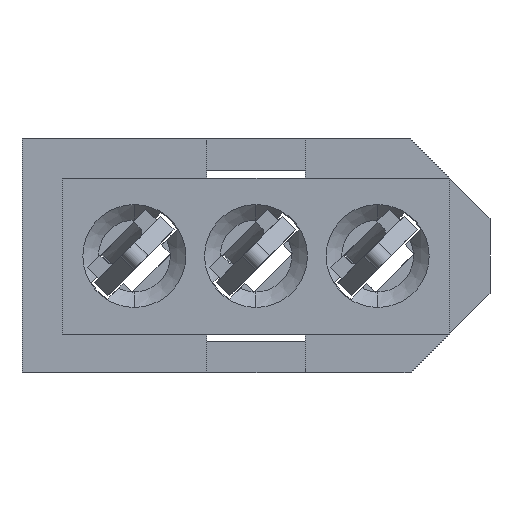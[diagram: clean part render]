
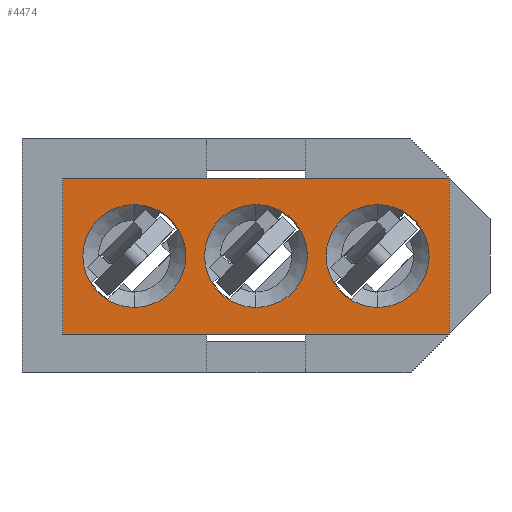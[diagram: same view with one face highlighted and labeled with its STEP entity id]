
A CAD part, front view. The second image highlights one B-rep face of the part: STEP entity #4474.
In plain terms, the highlighted planar face has unit normal (0, -1, 0).
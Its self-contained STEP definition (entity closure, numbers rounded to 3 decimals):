
#9 = EDGE_LOOP ( 'NONE', ( #2040, #771, #2001, #3821 ) ) ;
#65 = CARTESIAN_POINT ( 'NONE',  ( 0., -12.7, 0. ) ) ;
#254 = CARTESIAN_POINT ( 'NONE',  ( 3.962, -12.7, 1.676 ) ) ;
#388 = LINE ( 'NONE', #1455, #5583 ) ;
#542 = LINE ( 'NONE', #3797, #3066 ) ;
#565 = DIRECTION ( 'NONE',  ( 0., 0., 1. ) ) ;
#586 = AXIS2_PLACEMENT_3D ( 'NONE', #2626, #593, #5675 ) ;
#593 = DIRECTION ( 'NONE',  ( 0., 1., 0. ) ) ;
#771 = ORIENTED_EDGE ( 'NONE', *, *, #4602, .F. ) ;
#879 = DIRECTION ( 'NONE',  ( 1., 0., 0. ) ) ;
#964 = CARTESIAN_POINT ( 'NONE',  ( -2.324, -12.7, -2.54 ) ) ;
#1041 = FACE_BOUND ( 'NONE', #6220, .T. ) ;
#1257 = LINE ( 'NONE', #3853, #3906 ) ;
#1378 = AXIS2_PLACEMENT_3D ( 'NONE', #65, #4117, #565 ) ;
#1455 = CARTESIAN_POINT ( 'NONE',  ( -2.324, -12.7, -2.54 ) ) ;
#1521 = VERTEX_POINT ( 'NONE', #4332 ) ;
#1573 = EDGE_LOOP ( 'NONE', ( #3069, #2738 ) ) ;
#1607 = LINE ( 'NONE', #964, #5761 ) ;
#1710 = AXIS2_PLACEMENT_3D ( 'NONE', #2483, #3422, #2882 ) ;
#1718 = DIRECTION ( 'NONE',  ( 0., 0., 1. ) ) ;
#1769 = CIRCLE ( 'NONE', #2635, 1.676 ) ;
#1939 = PLANE ( 'NONE',  #6029 ) ;
#1948 = DIRECTION ( 'NONE',  ( -1., 0., 0. ) ) ;
#2001 = ORIENTED_EDGE ( 'NONE', *, *, #5042, .F. ) ;
#2040 = ORIENTED_EDGE ( 'NONE', *, *, #6297, .F. ) ;
#2057 = EDGE_LOOP ( 'NONE', ( #5653, #4884 ) ) ;
#2153 = FACE_BOUND ( 'NONE', #2057, .T. ) ;
#2242 = CIRCLE ( 'NONE', #2863, 1.676 ) ;
#2424 = DIRECTION ( 'NONE',  ( 0., 0., 1. ) ) ;
#2483 = CARTESIAN_POINT ( 'NONE',  ( 7.925, -12.7, 0. ) ) ;
#2559 = CARTESIAN_POINT ( 'NONE',  ( -2.324, -12.7, -2.54 ) ) ;
#2589 = EDGE_CURVE ( 'NONE', #5866, #1521, #1769, .T. ) ;
#2626 = CARTESIAN_POINT ( 'NONE',  ( 0., -12.7, 0. ) ) ;
#2635 = AXIS2_PLACEMENT_3D ( 'NONE', #3576, #3041, #4999 ) ;
#2738 = ORIENTED_EDGE ( 'NONE', *, *, #6352, .T. ) ;
#2773 = EDGE_CURVE ( 'NONE', #4012, #5973, #2242, .T. ) ;
#2781 = CARTESIAN_POINT ( 'NONE',  ( 0., -12.7, 1.676 ) ) ;
#2792 = CARTESIAN_POINT ( 'NONE',  ( 10.249, -12.7, -2.54 ) ) ;
#2863 = AXIS2_PLACEMENT_3D ( 'NONE', #5123, #5626, #1718 ) ;
#2882 = DIRECTION ( 'NONE',  ( 0., 0., 1. ) ) ;
#2941 = DIRECTION ( 'NONE',  ( 0., 0., 1. ) ) ;
#2960 = CARTESIAN_POINT ( 'NONE',  ( 3.962, -12.7, 0. ) ) ;
#2969 = VERTEX_POINT ( 'NONE', #4285 ) ;
#3041 = DIRECTION ( 'NONE',  ( 0., 1., 0. ) ) ;
#3066 = VECTOR ( 'NONE', #5298, 1000. ) ;
#3069 = ORIENTED_EDGE ( 'NONE', *, *, #5404, .T. ) ;
#3141 = ORIENTED_EDGE ( 'NONE', *, *, #3747, .T. ) ;
#3422 = DIRECTION ( 'NONE',  ( 0., 1., 0. ) ) ;
#3473 = CARTESIAN_POINT ( 'NONE',  ( 0., -12.7, -1.676 ) ) ;
#3576 = CARTESIAN_POINT ( 'NONE',  ( 7.925, -12.7, 0. ) ) ;
#3747 = EDGE_CURVE ( 'NONE', #1521, #5866, #4100, .T. ) ;
#3797 = CARTESIAN_POINT ( 'NONE',  ( 10.249, -12.7, -2.54 ) ) ;
#3821 = ORIENTED_EDGE ( 'NONE', *, *, #5600, .F. ) ;
#3853 = CARTESIAN_POINT ( 'NONE',  ( -2.324, -12.7, 2.54 ) ) ;
#3906 = VECTOR ( 'NONE', #879, 1000. ) ;
#4012 = VERTEX_POINT ( 'NONE', #254 ) ;
#4049 = DIRECTION ( 'NONE',  ( 0., 0., 1. ) ) ;
#4079 = CARTESIAN_POINT ( 'NONE',  ( 7.925, -12.7, 1.676 ) ) ;
#4100 = CIRCLE ( 'NONE', #1710, 1.676 ) ;
#4104 = VERTEX_POINT ( 'NONE', #2792 ) ;
#4117 = DIRECTION ( 'NONE',  ( 0., 1., 0. ) ) ;
#4285 = CARTESIAN_POINT ( 'NONE',  ( -2.324, -12.7, 2.54 ) ) ;
#4332 = CARTESIAN_POINT ( 'NONE',  ( 7.925, -12.7, -1.676 ) ) ;
#4474 = ADVANCED_FACE ( 'NONE', ( #1041, #2153, #5050, #4888 ), #1939, .F. ) ;
#4602 = EDGE_CURVE ( 'NONE', #4104, #6424, #388, .T. ) ;
#4883 = CARTESIAN_POINT ( 'NONE',  ( 0., -12.7, 0. ) ) ;
#4884 = ORIENTED_EDGE ( 'NONE', *, *, #6214, .T. ) ;
#4888 = FACE_OUTER_BOUND ( 'NONE', #9, .T. ) ;
#4999 = DIRECTION ( 'NONE',  ( 0., 0., 1. ) ) ;
#5042 = EDGE_CURVE ( 'NONE', #6289, #4104, #542, .T. ) ;
#5050 = FACE_BOUND ( 'NONE', #1573, .T. ) ;
#5123 = CARTESIAN_POINT ( 'NONE',  ( 3.962, -12.7, 0. ) ) ;
#5183 = VERTEX_POINT ( 'NONE', #2781 ) ;
#5217 = CIRCLE ( 'NONE', #5309, 1.676 ) ;
#5298 = DIRECTION ( 'NONE',  ( 0., 0., -1. ) ) ;
#5309 = AXIS2_PLACEMENT_3D ( 'NONE', #2960, #5506, #2941 ) ;
#5331 = CIRCLE ( 'NONE', #586, 1.676 ) ;
#5382 = DIRECTION ( 'NONE',  ( 0., 1., 0. ) ) ;
#5404 = EDGE_CURVE ( 'NONE', #5183, #6196, #5331, .T. ) ;
#5506 = DIRECTION ( 'NONE',  ( 0., 1., 0. ) ) ;
#5583 = VECTOR ( 'NONE', #1948, 1000. ) ;
#5597 = CARTESIAN_POINT ( 'NONE',  ( 10.249, -12.7, 2.54 ) ) ;
#5600 = EDGE_CURVE ( 'NONE', #2969, #6289, #1257, .T. ) ;
#5626 = DIRECTION ( 'NONE',  ( 0., 1., 0. ) ) ;
#5647 = CARTESIAN_POINT ( 'NONE',  ( 3.962, -12.7, -1.676 ) ) ;
#5653 = ORIENTED_EDGE ( 'NONE', *, *, #2773, .T. ) ;
#5675 = DIRECTION ( 'NONE',  ( 0., 0., 1. ) ) ;
#5761 = VECTOR ( 'NONE', #4049, 1000. ) ;
#5866 = VERTEX_POINT ( 'NONE', #4079 ) ;
#5973 = VERTEX_POINT ( 'NONE', #5647 ) ;
#5979 = ORIENTED_EDGE ( 'NONE', *, *, #2589, .T. ) ;
#6029 = AXIS2_PLACEMENT_3D ( 'NONE', #4883, #5382, #2424 ) ;
#6156 = CIRCLE ( 'NONE', #1378, 1.676 ) ;
#6196 = VERTEX_POINT ( 'NONE', #3473 ) ;
#6214 = EDGE_CURVE ( 'NONE', #5973, #4012, #5217, .T. ) ;
#6220 = EDGE_LOOP ( 'NONE', ( #5979, #3141 ) ) ;
#6289 = VERTEX_POINT ( 'NONE', #5597 ) ;
#6297 = EDGE_CURVE ( 'NONE', #6424, #2969, #1607, .T. ) ;
#6352 = EDGE_CURVE ( 'NONE', #6196, #5183, #6156, .T. ) ;
#6424 = VERTEX_POINT ( 'NONE', #2559 ) ;
